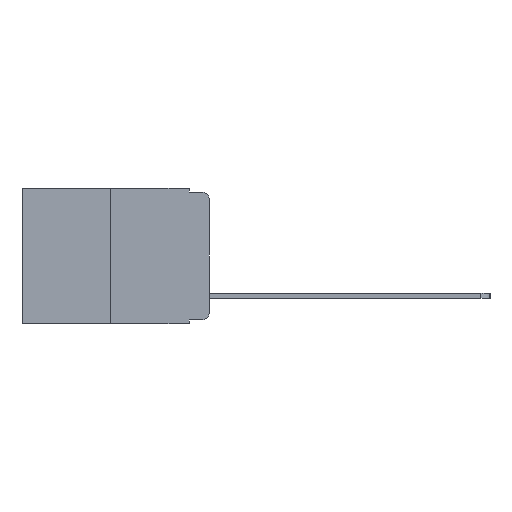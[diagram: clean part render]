
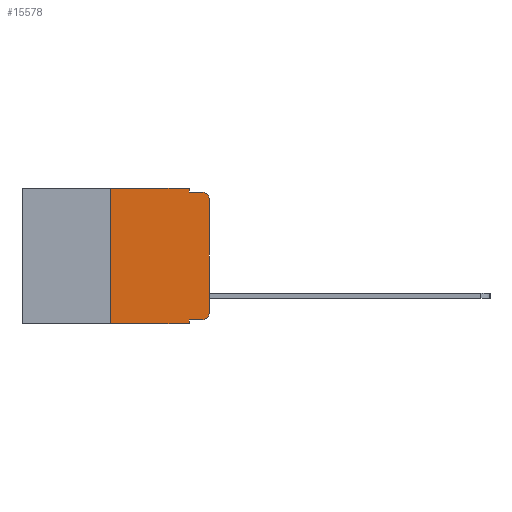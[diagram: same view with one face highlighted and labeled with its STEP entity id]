
A CAD part, left-side view. The second image highlights one B-rep face of the part: STEP entity #15578.
In plain terms, the highlighted planar face has unit normal (-1, 0, 0).
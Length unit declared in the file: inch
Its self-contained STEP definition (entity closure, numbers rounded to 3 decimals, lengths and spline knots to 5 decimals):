
#142 = VECTOR ( 'NONE', #3689, 39.37008 ) ;
#373 = ORIENTED_EDGE ( 'NONE', *, *, #1693, .F. ) ;
#488 = LINE ( 'NONE', #2896, #18214 ) ;
#609 = EDGE_CURVE ( 'NONE', #11131, #18377, #5046, .T. ) ;
#1482 = CARTESIAN_POINT ( 'NONE',  ( 0., 0.051, -0.343 ) ) ;
#1606 = CARTESIAN_POINT ( 'NONE',  ( 0., 0.473, 0. ) ) ;
#1653 = EDGE_CURVE ( 'NONE', #18481, #11131, #10686, .T. ) ;
#1693 = EDGE_CURVE ( 'NONE', #18481, #4699, #10137, .T. ) ;
#1697 = EDGE_CURVE ( 'NONE', #14314, #10514, #18210, .T. ) ;
#1702 = CARTESIAN_POINT ( 'NONE',  ( 0., 0.051, -0.333 ) ) ;
#1726 = EDGE_CURVE ( 'NONE', #9190, #14189, #4120, .T. ) ;
#1732 = EDGE_CURVE ( 'NONE', #14189, #6514, #13128, .T. ) ;
#1796 = EDGE_CURVE ( 'NONE', #18777, #6514, #16646, .T. ) ;
#1829 = EDGE_CURVE ( 'NONE', #18377, #18777, #19968, .T. ) ;
#2748 = CARTESIAN_POINT ( 'NONE',  ( 0., 0.051, -0.01 ) ) ;
#2758 = AXIS2_PLACEMENT_3D ( 'NONE', #1606, #10710, #22443 ) ;
#2846 = EDGE_CURVE ( 'NONE', #10514, #9190, #18936, .T. ) ;
#2896 = CARTESIAN_POINT ( 'NONE',  ( 0., 0.473, -0.343 ) ) ;
#2958 = DIRECTION ( 'NONE',  ( 0., -1., 0. ) ) ;
#3402 = PLANE ( 'NONE',  #2758 ) ;
#3689 = DIRECTION ( 'NONE',  ( 0., -1., 0. ) ) ;
#4000 = ORIENTED_EDGE ( 'NONE', *, *, #8025, .T. ) ;
#4120 = LINE ( 'NONE', #13207, #8433 ) ;
#4306 = CARTESIAN_POINT ( 'NONE',  ( 0., 0.02, -0.313 ) ) ;
#4333 = DIRECTION ( 'NONE',  ( -1., 0., 0. ) ) ;
#4358 = DIRECTION ( 'NONE',  ( 0., 0., -1. ) ) ;
#4699 = VERTEX_POINT ( 'NONE', #1482 ) ;
#5046 = CIRCLE ( 'NONE', #5215, 0.02 ) ;
#5215 = AXIS2_PLACEMENT_3D ( 'NONE', #4306, #4333, #4358 ) ;
#5447 = ORIENTED_EDGE ( 'NONE', *, *, #609, .T. ) ;
#5733 = CARTESIAN_POINT ( 'NONE',  ( 0., 0.02, -0.333 ) ) ;
#5775 = ORIENTED_EDGE ( 'NONE', *, *, #1796, .T. ) ;
#6514 = VERTEX_POINT ( 'NONE', #8093 ) ;
#7142 = ORIENTED_EDGE ( 'NONE', *, *, #1829, .T. ) ;
#7244 = CARTESIAN_POINT ( 'NONE',  ( 0., 0.473, 0. ) ) ;
#7512 = EDGE_LOOP ( 'NONE', ( #7142, #5775, #14791, #11074, #10043, #15491, #4000, #373, #10399, #5447 ) ) ;
#8025 = EDGE_CURVE ( 'NONE', #14314, #4699, #488, .T. ) ;
#8093 = CARTESIAN_POINT ( 'NONE',  ( 0., 0.02, -0.01 ) ) ;
#8433 = VECTOR ( 'NONE', #13671, 39.37008 ) ;
#9017 = VECTOR ( 'NONE', #22380, 39.37008 ) ;
#9190 = VERTEX_POINT ( 'NONE', #17860 ) ;
#10043 = ORIENTED_EDGE ( 'NONE', *, *, #2846, .F. ) ;
#10137 = LINE ( 'NONE', #13054, #9017 ) ;
#10372 = CARTESIAN_POINT ( 'NONE',  ( 0., 0.25, -0.343 ) ) ;
#10399 = ORIENTED_EDGE ( 'NONE', *, *, #1653, .T. ) ;
#10514 = VERTEX_POINT ( 'NONE', #22307 ) ;
#10686 = LINE ( 'NONE', #14216, #19245 ) ;
#10710 = DIRECTION ( 'NONE',  ( 1., 0., 0. ) ) ;
#11074 = ORIENTED_EDGE ( 'NONE', *, *, #1726, .F. ) ;
#11131 = VERTEX_POINT ( 'NONE', #5733 ) ;
#11428 = DIRECTION ( 'NONE',  ( 0., 0., 1. ) ) ;
#13026 = CARTESIAN_POINT ( 'NONE',  ( 0., 0.02, -0.03 ) ) ;
#13054 = CARTESIAN_POINT ( 'NONE',  ( 0., 0.051, 0. ) ) ;
#13128 = LINE ( 'NONE', #19876, #21515 ) ;
#13207 = CARTESIAN_POINT ( 'NONE',  ( 0., 0.051, 0. ) ) ;
#13462 = DIRECTION ( 'NONE',  ( 0., -1., 0. ) ) ;
#13671 = DIRECTION ( 'NONE',  ( 0., 0., -1. ) ) ;
#13910 = CARTESIAN_POINT ( 'NONE',  ( 0., 0., -0.313 ) ) ;
#14189 = VERTEX_POINT ( 'NONE', #2748 ) ;
#14216 = CARTESIAN_POINT ( 'NONE',  ( 0., 0.051, -0.333 ) ) ;
#14314 = VERTEX_POINT ( 'NONE', #10372 ) ;
#14330 = AXIS2_PLACEMENT_3D ( 'NONE', #13026, #20043, #22167 ) ;
#14791 = ORIENTED_EDGE ( 'NONE', *, *, #1732, .F. ) ;
#15491 = ORIENTED_EDGE ( 'NONE', *, *, #1697, .F. ) ;
#15578 = ADVANCED_FACE ( 'NONE', ( #21490 ), #3402, .F. ) ;
#15582 = VECTOR ( 'NONE', #18573, 39.37008 ) ;
#16617 = CARTESIAN_POINT ( 'NONE',  ( 0., 0., -0.03 ) ) ;
#16646 = CIRCLE ( 'NONE', #14330, 0.02 ) ;
#17239 = DIRECTION ( 'NONE',  ( 0., -1., 0. ) ) ;
#17860 = CARTESIAN_POINT ( 'NONE',  ( 0., 0.051, 0. ) ) ;
#18210 = LINE ( 'NONE', #22327, #21991 ) ;
#18214 = VECTOR ( 'NONE', #2958, 39.37008 ) ;
#18377 = VERTEX_POINT ( 'NONE', #13910 ) ;
#18481 = VERTEX_POINT ( 'NONE', #1702 ) ;
#18573 = DIRECTION ( 'NONE',  ( 0., 0., 1. ) ) ;
#18777 = VERTEX_POINT ( 'NONE', #16617 ) ;
#18936 = LINE ( 'NONE', #7244, #142 ) ;
#19245 = VECTOR ( 'NONE', #17239, 39.37008 ) ;
#19700 = CARTESIAN_POINT ( 'NONE',  ( 0., 0., 0. ) ) ;
#19876 = CARTESIAN_POINT ( 'NONE',  ( 0., 0.051, -0.01 ) ) ;
#19968 = LINE ( 'NONE', #19700, #15582 ) ;
#20043 = DIRECTION ( 'NONE',  ( -1., 0., 0. ) ) ;
#21490 = FACE_OUTER_BOUND ( 'NONE', #7512, .T. ) ;
#21515 = VECTOR ( 'NONE', #13462, 39.37008 ) ;
#21991 = VECTOR ( 'NONE', #11428, 39.37008 ) ;
#22167 = DIRECTION ( 'NONE',  ( 0., 0., -1. ) ) ;
#22307 = CARTESIAN_POINT ( 'NONE',  ( 0., 0.25, 0. ) ) ;
#22327 = CARTESIAN_POINT ( 'NONE',  ( 0., 0.25, 0. ) ) ;
#22380 = DIRECTION ( 'NONE',  ( 0., 0., -1. ) ) ;
#22443 = DIRECTION ( 'NONE',  ( 0., 0., -1. ) ) ;
